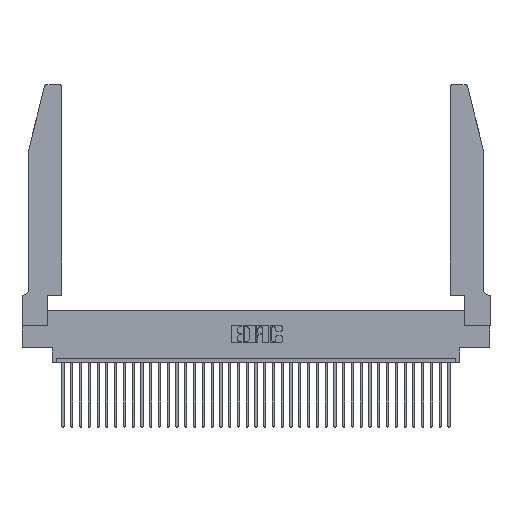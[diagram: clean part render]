
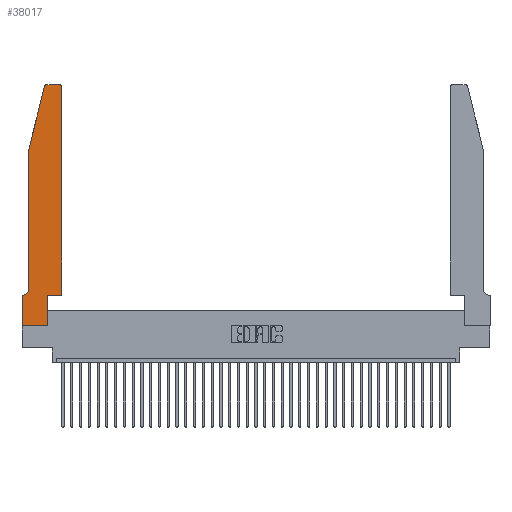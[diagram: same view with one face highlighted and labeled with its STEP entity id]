
A CAD part, top view. The second image highlights one B-rep face of the part: STEP entity #38017.
In plain terms, the highlighted planar face has unit normal (0, 0, 1).
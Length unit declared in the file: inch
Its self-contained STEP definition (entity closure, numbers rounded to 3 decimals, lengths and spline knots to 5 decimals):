
#429 = CARTESIAN_POINT ( 'NONE',  ( 0., 0., 0.37 ) ) ;
#1023 = ORIENTED_EDGE ( 'NONE', *, *, #20635, .T. ) ;
#1146 = VECTOR ( 'NONE', #15196, 39.37008 ) ;
#1487 = EDGE_CURVE ( 'NONE', #20808, #13110, #2983, .T. ) ;
#1618 = AXIS2_PLACEMENT_3D ( 'NONE', #27446, #33374, #27302 ) ;
#2090 = VERTEX_POINT ( 'NONE', #9399 ) ;
#2210 = DIRECTION ( 'NONE',  ( 0., -1., 0. ) ) ;
#2404 = DIRECTION ( 'NONE',  ( 0., 1., 0. ) ) ;
#2557 = CARTESIAN_POINT ( 'NONE',  ( 0.0055, 0.35, 0.37 ) ) ;
#2983 = LINE ( 'NONE', #9705, #34922 ) ;
#3111 = CARTESIAN_POINT ( 'NONE',  ( 0.4505, 2.72, 0.37 ) ) ;
#3151 = LINE ( 'NONE', #4899, #10146 ) ;
#4204 = AXIS2_PLACEMENT_3D ( 'NONE', #5592, #31861, #14298 ) ;
#4313 = ORIENTED_EDGE ( 'NONE', *, *, #25931, .T. ) ;
#4428 = CIRCLE ( 'NONE', #1618, 0.03 ) ;
#4439 = LINE ( 'NONE', #26813, #1146 ) ;
#4899 = CARTESIAN_POINT ( 'NONE',  ( 0.2865, 0.35, 0.37 ) ) ;
#5426 = CARTESIAN_POINT ( 'NONE',  ( 0.4505, 0.35, 0.37 ) ) ;
#5592 = CARTESIAN_POINT ( 'NONE',  ( 0., 0.35, 0.37 ) ) ;
#6527 = CARTESIAN_POINT ( 'NONE',  ( 0.0055, 0.42, 0.37 ) ) ;
#6645 = VECTOR ( 'NONE', #8102, 39.37008 ) ;
#7041 = EDGE_CURVE ( 'NONE', #34359, #20808, #3151, .T. ) ;
#7264 = LINE ( 'NONE', #28789, #12305 ) ;
#8102 = DIRECTION ( 'NONE',  ( -0.239, -0.971, 0. ) ) ;
#8412 = LINE ( 'NONE', #429, #16744 ) ;
#8798 = LINE ( 'NONE', #18860, #32374 ) ;
#9114 = EDGE_CURVE ( 'NONE', #26539, #2090, #4428, .T. ) ;
#9192 = CARTESIAN_POINT ( 'NONE',  ( 0.0755, 0.35, 0.37 ) ) ;
#9399 = CARTESIAN_POINT ( 'NONE',  ( 0.25487, 2.72718, 0.37 ) ) ;
#9701 = CARTESIAN_POINT ( 'NONE',  ( 0.2865, 0.35, 0.37 ) ) ;
#9705 = CARTESIAN_POINT ( 'NONE',  ( 0.4505, 0.35, 0.37 ) ) ;
#9877 = EDGE_CURVE ( 'NONE', #2090, #17936, #12196, .T. ) ;
#10146 = VECTOR ( 'NONE', #2404, 39.37008 ) ;
#12196 = LINE ( 'NONE', #25554, #6645 ) ;
#12305 = VECTOR ( 'NONE', #2210, 39.37008 ) ;
#12610 = ORIENTED_EDGE ( 'NONE', *, *, #9877, .T. ) ;
#12811 = LINE ( 'NONE', #26969, #32239 ) ;
#13041 = CIRCLE ( 'NONE', #36289, 0.03 ) ;
#13110 = VERTEX_POINT ( 'NONE', #5426 ) ;
#14298 = DIRECTION ( 'NONE',  ( 1., 0., 0. ) ) ;
#14890 = CARTESIAN_POINT ( 'NONE',  ( 0., 0.35, 0.37 ) ) ;
#15196 = DIRECTION ( 'NONE',  ( 0., -1., 0. ) ) ;
#16371 = CIRCLE ( 'NONE', #29979, 0.07 ) ;
#16744 = VECTOR ( 'NONE', #30122, 39.37008 ) ;
#17103 = EDGE_CURVE ( 'NONE', #32763, #18294, #7264, .T. ) ;
#17302 = CARTESIAN_POINT ( 'NONE',  ( 0.284, 2.75, 0.37 ) ) ;
#17691 = CARTESIAN_POINT ( 'NONE',  ( 0.4205, 2.72, 0.37 ) ) ;
#17936 = VERTEX_POINT ( 'NONE', #37617 ) ;
#18039 = DIRECTION ( 'NONE',  ( 0., 0., 1. ) ) ;
#18135 = VERTEX_POINT ( 'NONE', #28204 ) ;
#18294 = VERTEX_POINT ( 'NONE', #33446 ) ;
#18352 = VECTOR ( 'NONE', #29761, 39.37008 ) ;
#18499 = DIRECTION ( 'NONE',  ( 1., 0., 0. ) ) ;
#18860 = CARTESIAN_POINT ( 'NONE',  ( 0.4505, 0.35, 0.37 ) ) ;
#19385 = DIRECTION ( 'NONE',  ( 0., 1., 0. ) ) ;
#19389 = VERTEX_POINT ( 'NONE', #3111 ) ;
#19698 = ORIENTED_EDGE ( 'NONE', *, *, #23397, .T. ) ;
#20540 = DIRECTION ( 'NONE',  ( 1., 0., 0. ) ) ;
#20635 = EDGE_CURVE ( 'NONE', #18294, #34359, #8412, .T. ) ;
#20808 = VERTEX_POINT ( 'NONE', #9701 ) ;
#21245 = CARTESIAN_POINT ( 'NONE',  ( 0.2865, 0., 0.37 ) ) ;
#21842 = EDGE_CURVE ( 'NONE', #18135, #32635, #16371, .T. ) ;
#22973 = PLANE ( 'NONE',  #4204 ) ;
#23397 = EDGE_CURVE ( 'NONE', #13110, #19389, #8798, .T. ) ;
#23702 = ORIENTED_EDGE ( 'NONE', *, *, #9114, .T. ) ;
#25554 = CARTESIAN_POINT ( 'NONE',  ( 0.0755, 2., 0.37 ) ) ;
#25931 = EDGE_CURVE ( 'NONE', #34701, #26539, #12811, .T. ) ;
#26027 = ORIENTED_EDGE ( 'NONE', *, *, #21842, .T. ) ;
#26539 = VERTEX_POINT ( 'NONE', #17302 ) ;
#26813 = CARTESIAN_POINT ( 'NONE',  ( 0.0755, 2., 0.37 ) ) ;
#26969 = CARTESIAN_POINT ( 'NONE',  ( 0.2605, 2.75, 0.37 ) ) ;
#27302 = DIRECTION ( 'NONE',  ( 1., 0., 0. ) ) ;
#27437 = EDGE_LOOP ( 'NONE', ( #4313, #23702, #12610, #30511, #26027, #34741, #31838, #1023, #37825, #35084, #19698, #29401 ) ) ;
#27446 = CARTESIAN_POINT ( 'NONE',  ( 0.284, 2.72, 0.37 ) ) ;
#28204 = CARTESIAN_POINT ( 'NONE',  ( 0.0755, 0.42, 0.37 ) ) ;
#28789 = CARTESIAN_POINT ( 'NONE',  ( 0., 0., 0.37 ) ) ;
#29401 = ORIENTED_EDGE ( 'NONE', *, *, #34260, .T. ) ;
#29761 = DIRECTION ( 'NONE',  ( -1., 0., 0. ) ) ;
#29979 = AXIS2_PLACEMENT_3D ( 'NONE', #6527, #30478, #30622 ) ;
#30122 = DIRECTION ( 'NONE',  ( 1., 0., 0. ) ) ;
#30355 = EDGE_CURVE ( 'NONE', #32635, #32763, #35025, .T. ) ;
#30478 = DIRECTION ( 'NONE',  ( 0., 0., -1. ) ) ;
#30511 = ORIENTED_EDGE ( 'NONE', *, *, #31781, .T. ) ;
#30622 = DIRECTION ( 'NONE',  ( -1., 0., 0. ) ) ;
#31781 = EDGE_CURVE ( 'NONE', #17936, #18135, #4439, .T. ) ;
#31838 = ORIENTED_EDGE ( 'NONE', *, *, #17103, .T. ) ;
#31861 = DIRECTION ( 'NONE',  ( 0., 0., 1. ) ) ;
#32239 = VECTOR ( 'NONE', #32888, 39.37008 ) ;
#32374 = VECTOR ( 'NONE', #19385, 39.37008 ) ;
#32635 = VERTEX_POINT ( 'NONE', #2557 ) ;
#32763 = VERTEX_POINT ( 'NONE', #14890 ) ;
#32888 = DIRECTION ( 'NONE',  ( -1., 0., 0. ) ) ;
#33374 = DIRECTION ( 'NONE',  ( 0., 0., 1. ) ) ;
#33446 = CARTESIAN_POINT ( 'NONE',  ( 0., 0., 0.37 ) ) ;
#34260 = EDGE_CURVE ( 'NONE', #19389, #34701, #13041, .T. ) ;
#34359 = VERTEX_POINT ( 'NONE', #21245 ) ;
#34701 = VERTEX_POINT ( 'NONE', #37801 ) ;
#34741 = ORIENTED_EDGE ( 'NONE', *, *, #30355, .T. ) ;
#34922 = VECTOR ( 'NONE', #18499, 39.37008 ) ;
#35025 = LINE ( 'NONE', #9192, #18352 ) ;
#35084 = ORIENTED_EDGE ( 'NONE', *, *, #1487, .T. ) ;
#35408 = FACE_OUTER_BOUND ( 'NONE', #27437, .T. ) ;
#36289 = AXIS2_PLACEMENT_3D ( 'NONE', #17691, #18039, #20540 ) ;
#37617 = CARTESIAN_POINT ( 'NONE',  ( 0.0755, 2., 0.37 ) ) ;
#37801 = CARTESIAN_POINT ( 'NONE',  ( 0.4205, 2.75, 0.37 ) ) ;
#37825 = ORIENTED_EDGE ( 'NONE', *, *, #7041, .T. ) ;
#38017 = ADVANCED_FACE ( 'NONE', ( #35408 ), #22973, .T. ) ;
